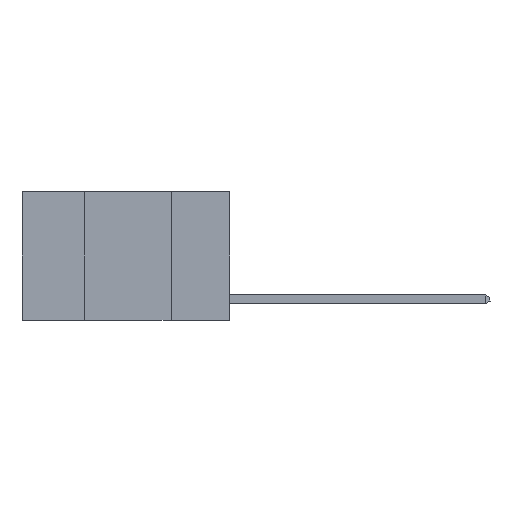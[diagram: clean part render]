
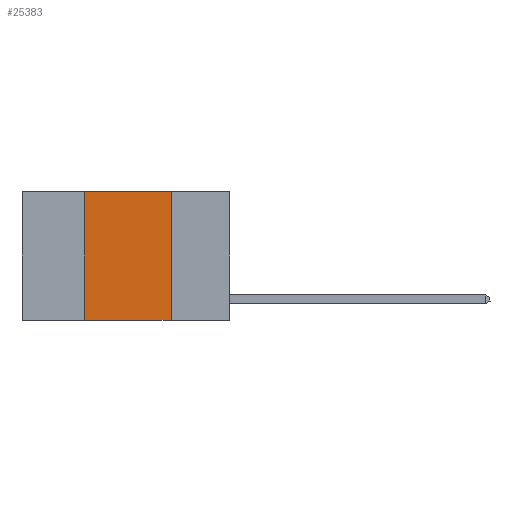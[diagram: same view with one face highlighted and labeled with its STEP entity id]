
A CAD part, left-side view. The second image highlights one B-rep face of the part: STEP entity #25383.
In plain terms, the highlighted planar face has unit normal (-1, 0, 0).
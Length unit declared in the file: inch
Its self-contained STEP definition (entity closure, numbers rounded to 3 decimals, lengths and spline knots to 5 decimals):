
#805 = DIRECTION ( 'NONE',  ( 1., 0., 0. ) ) ;
#1463 = EDGE_CURVE ( 'NONE', #21875, #25430, #3866, .T. ) ;
#2028 = VERTEX_POINT ( 'NONE', #19507 ) ;
#3866 = LINE ( 'NONE', #11734, #18441 ) ;
#5057 = DIRECTION ( 'NONE',  ( 0., -1., 0. ) ) ;
#5949 = CARTESIAN_POINT ( 'NONE',  ( 0., 0.6, 0. ) ) ;
#6261 = AXIS2_PLACEMENT_3D ( 'NONE', #27284, #805, #16252 ) ;
#7716 = CARTESIAN_POINT ( 'NONE',  ( 0., 0.17, 0. ) ) ;
#8171 = CARTESIAN_POINT ( 'NONE',  ( 0., 0.42, -0.37 ) ) ;
#8252 = VERTEX_POINT ( 'NONE', #11794 ) ;
#8272 = EDGE_CURVE ( 'NONE', #8252, #2028, #21854, .T. ) ;
#11273 = ORIENTED_EDGE ( 'NONE', *, *, #20755, .F. ) ;
#11734 = CARTESIAN_POINT ( 'NONE',  ( 0., 0.42, 0. ) ) ;
#11794 = CARTESIAN_POINT ( 'NONE',  ( 0., 0.17, 0. ) ) ;
#12337 = EDGE_CURVE ( 'NONE', #21875, #2028, #23658, .T. ) ;
#13656 = FACE_OUTER_BOUND ( 'NONE', #27850, .T. ) ;
#13849 = ORIENTED_EDGE ( 'NONE', *, *, #12337, .T. ) ;
#14311 = VECTOR ( 'NONE', #5057, 39.37008 ) ;
#16089 = ORIENTED_EDGE ( 'NONE', *, *, #1463, .F. ) ;
#16252 = DIRECTION ( 'NONE',  ( 0., 0., -1. ) ) ;
#18224 = DIRECTION ( 'NONE',  ( 0., 0., 1. ) ) ;
#18441 = VECTOR ( 'NONE', #18224, 39.37008 ) ;
#19507 = CARTESIAN_POINT ( 'NONE',  ( 0., 0.17, -0.37 ) ) ;
#20104 = LINE ( 'NONE', #5949, #26660 ) ;
#20755 = EDGE_CURVE ( 'NONE', #25430, #8252, #20104, .T. ) ;
#21377 = ORIENTED_EDGE ( 'NONE', *, *, #8272, .F. ) ;
#21854 = LINE ( 'NONE', #7716, #28049 ) ;
#21875 = VERTEX_POINT ( 'NONE', #8171 ) ;
#22738 = PLANE ( 'NONE',  #6261 ) ;
#22913 = DIRECTION ( 'NONE',  ( 0., 0., -1. ) ) ;
#23658 = LINE ( 'NONE', #25127, #14311 ) ;
#23665 = DIRECTION ( 'NONE',  ( 0., -1., 0. ) ) ;
#25127 = CARTESIAN_POINT ( 'NONE',  ( 0., 0.6, -0.37 ) ) ;
#25342 = CARTESIAN_POINT ( 'NONE',  ( 0., 0.42, 0. ) ) ;
#25383 = ADVANCED_FACE ( 'NONE', ( #13656 ), #22738, .F. ) ;
#25430 = VERTEX_POINT ( 'NONE', #25342 ) ;
#26660 = VECTOR ( 'NONE', #23665, 39.37008 ) ;
#27284 = CARTESIAN_POINT ( 'NONE',  ( 0., 0.6, 0. ) ) ;
#27850 = EDGE_LOOP ( 'NONE', ( #21377, #11273, #16089, #13849 ) ) ;
#28049 = VECTOR ( 'NONE', #22913, 39.37008 ) ;
